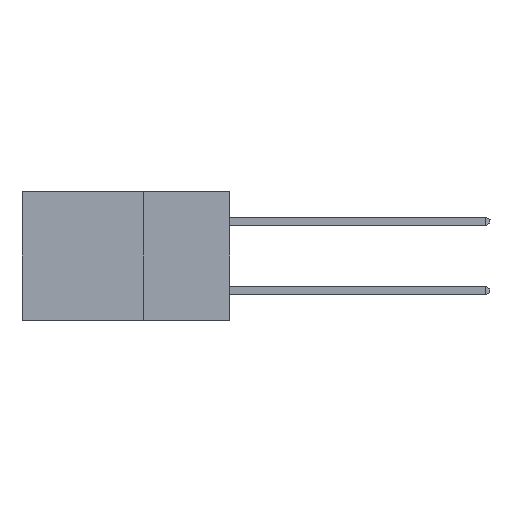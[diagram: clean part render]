
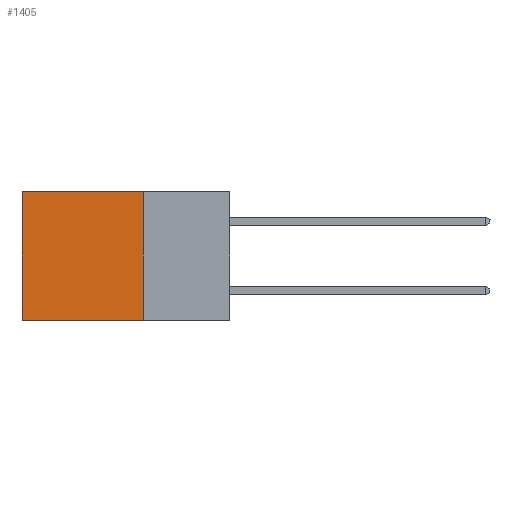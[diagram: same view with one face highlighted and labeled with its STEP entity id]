
A CAD part, left-side view. The second image highlights one B-rep face of the part: STEP entity #1405.
In plain terms, the highlighted planar face has unit normal (-1, 0, 0).
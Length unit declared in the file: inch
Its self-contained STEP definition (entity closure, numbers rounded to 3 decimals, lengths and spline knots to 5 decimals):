
#569 = CARTESIAN_POINT ( 'NONE',  ( 0.298, 0.25, -0.37 ) ) ;
#652 = PLANE ( 'NONE',  #5333 ) ;
#874 = VECTOR ( 'NONE', #4695, 39.37008 ) ;
#1342 = EDGE_CURVE ( 'NONE', #8935, #12788, #12299, .T. ) ;
#1405 = ADVANCED_FACE ( 'NONE', ( #7791 ), #652, .F. ) ;
#1522 = ORIENTED_EDGE ( 'NONE', *, *, #5949, .F. ) ;
#2048 = DIRECTION ( 'NONE',  ( 1., 0., 0. ) ) ;
#3683 = CARTESIAN_POINT ( 'NONE',  ( 0.298, 0.6, 0. ) ) ;
#4215 = VECTOR ( 'NONE', #11125, 39.37008 ) ;
#4695 = DIRECTION ( 'NONE',  ( 0., 0., -1. ) ) ;
#4797 = ORIENTED_EDGE ( 'NONE', *, *, #9924, .T. ) ;
#5333 = AXIS2_PLACEMENT_3D ( 'NONE', #18854, #2048, #14200 ) ;
#5949 = EDGE_CURVE ( 'NONE', #8426, #14693, #11408, .T. ) ;
#5973 = LINE ( 'NONE', #8618, #8122 ) ;
#7791 = FACE_OUTER_BOUND ( 'NONE', #14916, .T. ) ;
#7882 = CARTESIAN_POINT ( 'NONE',  ( 0.298, 0.25, 0. ) ) ;
#8122 = VECTOR ( 'NONE', #13085, 39.37008 ) ;
#8426 = VERTEX_POINT ( 'NONE', #18533 ) ;
#8618 = CARTESIAN_POINT ( 'NONE',  ( 0.298, 0.25, 0. ) ) ;
#8935 = VERTEX_POINT ( 'NONE', #7882 ) ;
#9924 = EDGE_CURVE ( 'NONE', #12788, #14693, #13934, .T. ) ;
#9979 = VECTOR ( 'NONE', #14248, 39.37008 ) ;
#10347 = CARTESIAN_POINT ( 'NONE',  ( 0.298, 0.6, -0.37 ) ) ;
#11125 = DIRECTION ( 'NONE',  ( 0., 1., 0. ) ) ;
#11190 = CARTESIAN_POINT ( 'NONE',  ( 0.298, 0.25, 0. ) ) ;
#11408 = LINE ( 'NONE', #569, #9979 ) ;
#12299 = LINE ( 'NONE', #11190, #4215 ) ;
#12788 = VERTEX_POINT ( 'NONE', #3683 ) ;
#13085 = DIRECTION ( 'NONE',  ( 0., 0., -1. ) ) ;
#13934 = LINE ( 'NONE', #15311, #874 ) ;
#14200 = DIRECTION ( 'NONE',  ( 0., 0., -1. ) ) ;
#14248 = DIRECTION ( 'NONE',  ( 0., 1., 0. ) ) ;
#14693 = VERTEX_POINT ( 'NONE', #10347 ) ;
#14916 = EDGE_LOOP ( 'NONE', ( #4797, #1522, #16225, #16072 ) ) ;
#15311 = CARTESIAN_POINT ( 'NONE',  ( 0.298, 0.6, 0. ) ) ;
#16072 = ORIENTED_EDGE ( 'NONE', *, *, #1342, .T. ) ;
#16225 = ORIENTED_EDGE ( 'NONE', *, *, #16497, .F. ) ;
#16497 = EDGE_CURVE ( 'NONE', #8935, #8426, #5973, .T. ) ;
#18533 = CARTESIAN_POINT ( 'NONE',  ( 0.298, 0.25, -0.37 ) ) ;
#18854 = CARTESIAN_POINT ( 'NONE',  ( 0.298, 0.25, 0. ) ) ;
